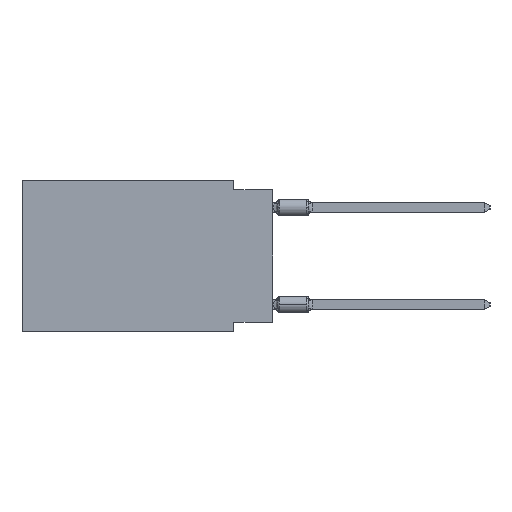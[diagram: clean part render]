
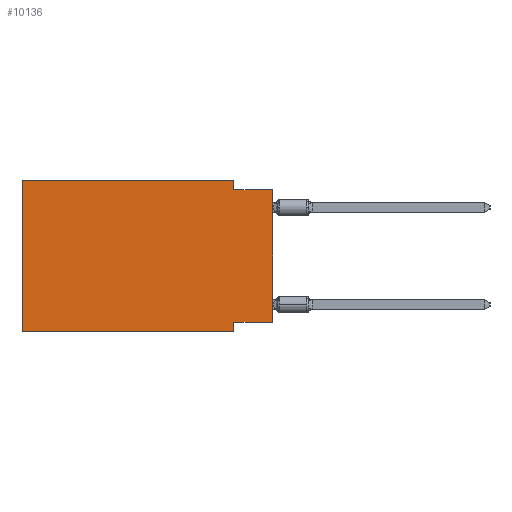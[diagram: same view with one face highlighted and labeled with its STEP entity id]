
A CAD part, left-side view. The second image highlights one B-rep face of the part: STEP entity #10136.
In plain terms, the highlighted planar face has unit normal (-1, 0, 0).
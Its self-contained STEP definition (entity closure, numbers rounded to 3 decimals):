
#2403 = EDGE_CURVE ( 'NONE', #34300, #35724, #3227, .T. ) ;
#3074 = PLANE ( 'NONE',  #36051 ) ;
#3227 = LINE ( 'NONE', #15440, #22596 ) ;
#3303 = VERTEX_POINT ( 'NONE', #22707 ) ;
#3503 = ORIENTED_EDGE ( 'NONE', *, *, #7575, .F. ) ;
#4296 = CARTESIAN_POINT ( 'NONE',  ( 0., 0., -0.635 ) ) ;
#6061 = VECTOR ( 'NONE', #17553, 1000. ) ;
#7575 = EDGE_CURVE ( 'NONE', #7789, #28297, #34504, .T. ) ;
#7760 = DIRECTION ( 'NONE',  ( 0., 1., 0. ) ) ;
#7789 = VERTEX_POINT ( 'NONE', #24601 ) ;
#9478 = DIRECTION ( 'NONE',  ( 0., 0., -1. ) ) ;
#10136 = ADVANCED_FACE ( 'NONE', ( #36728 ), #3074, .F. ) ;
#10223 = VECTOR ( 'NONE', #7760, 1000. ) ;
#11409 = CARTESIAN_POINT ( 'NONE',  ( 0., 0., 0. ) ) ;
#11563 = ORIENTED_EDGE ( 'NONE', *, *, #27276, .F. ) ;
#11667 = VECTOR ( 'NONE', #11803, 1000. ) ;
#11803 = DIRECTION ( 'NONE',  ( 0., 0., 1. ) ) ;
#13153 = ORIENTED_EDGE ( 'NONE', *, *, #30991, .F. ) ;
#14601 = DIRECTION ( 'NONE',  ( 0., -1., 0. ) ) ;
#15440 = CARTESIAN_POINT ( 'NONE',  ( 0., 16.383, 0. ) ) ;
#17553 = DIRECTION ( 'NONE',  ( 0., 0., 1. ) ) ;
#17715 = DIRECTION ( 'NONE',  ( 0., 0., -1. ) ) ;
#17812 = LINE ( 'NONE', #11409, #11667 ) ;
#18923 = CARTESIAN_POINT ( 'NONE',  ( 0., 16.383, -9.906 ) ) ;
#19049 = EDGE_CURVE ( 'NONE', #3303, #7789, #28595, .T. ) ;
#19502 = CARTESIAN_POINT ( 'NONE',  ( 0., 2.54, -9.906 ) ) ;
#19575 = CARTESIAN_POINT ( 'NONE',  ( 0., 0., -9.271 ) ) ;
#20283 = CARTESIAN_POINT ( 'NONE',  ( 0., 16.383, 0. ) ) ;
#20341 = ORIENTED_EDGE ( 'NONE', *, *, #38689, .T. ) ;
#21105 = CARTESIAN_POINT ( 'NONE',  ( 0., 16.383, 0. ) ) ;
#21248 = EDGE_CURVE ( 'NONE', #29459, #31257, #23619, .T. ) ;
#21683 = CARTESIAN_POINT ( 'NONE',  ( 0., 2.54, -9.906 ) ) ;
#22413 = EDGE_CURVE ( 'NONE', #3303, #31257, #17812, .T. ) ;
#22596 = VECTOR ( 'NONE', #36303, 1000. ) ;
#22707 = CARTESIAN_POINT ( 'NONE',  ( 0., 0., -9.271 ) ) ;
#23619 = LINE ( 'NONE', #35842, #27612 ) ;
#23967 = CARTESIAN_POINT ( 'NONE',  ( 0., 16.383, 0. ) ) ;
#24601 = CARTESIAN_POINT ( 'NONE',  ( 0., 2.54, -9.271 ) ) ;
#25936 = VERTEX_POINT ( 'NONE', #34631 ) ;
#26079 = CARTESIAN_POINT ( 'NONE',  ( 0., 2.54, 0. ) ) ;
#26273 = DIRECTION ( 'NONE',  ( 0., 0., -1. ) ) ;
#26600 = VECTOR ( 'NONE', #9478, 1000. ) ;
#26767 = LINE ( 'NONE', #18923, #34926 ) ;
#27276 = EDGE_CURVE ( 'NONE', #35724, #29459, #34892, .T. ) ;
#27612 = VECTOR ( 'NONE', #14601, 1000. ) ;
#27640 = ORIENTED_EDGE ( 'NONE', *, *, #2403, .F. ) ;
#28297 = VERTEX_POINT ( 'NONE', #19502 ) ;
#28595 = LINE ( 'NONE', #19575, #10223 ) ;
#28654 = ORIENTED_EDGE ( 'NONE', *, *, #22413, .T. ) ;
#29389 = ORIENTED_EDGE ( 'NONE', *, *, #21248, .F. ) ;
#29459 = VERTEX_POINT ( 'NONE', #30021 ) ;
#30021 = CARTESIAN_POINT ( 'NONE',  ( 0., 2.54, -0.635 ) ) ;
#30951 = DIRECTION ( 'NONE',  ( 0., -1., 0. ) ) ;
#30991 = EDGE_CURVE ( 'NONE', #25936, #34300, #36766, .T. ) ;
#31257 = VERTEX_POINT ( 'NONE', #4296 ) ;
#33527 = DIRECTION ( 'NONE',  ( 1., 0., 0. ) ) ;
#34300 = VERTEX_POINT ( 'NONE', #20283 ) ;
#34504 = LINE ( 'NONE', #21683, #26600 ) ;
#34631 = CARTESIAN_POINT ( 'NONE',  ( 0., 16.383, -9.906 ) ) ;
#34892 = LINE ( 'NONE', #26079, #37302 ) ;
#34926 = VECTOR ( 'NONE', #30951, 1000. ) ;
#35724 = VERTEX_POINT ( 'NONE', #37093 ) ;
#35842 = CARTESIAN_POINT ( 'NONE',  ( 0., 0., -0.635 ) ) ;
#36051 = AXIS2_PLACEMENT_3D ( 'NONE', #21105, #33527, #17715 ) ;
#36303 = DIRECTION ( 'NONE',  ( 0., -1., 0. ) ) ;
#36728 = FACE_OUTER_BOUND ( 'NONE', #37600, .T. ) ;
#36766 = LINE ( 'NONE', #23967, #6061 ) ;
#37093 = CARTESIAN_POINT ( 'NONE',  ( 0., 2.54, 0. ) ) ;
#37302 = VECTOR ( 'NONE', #26273, 1000. ) ;
#37600 = EDGE_LOOP ( 'NONE', ( #28654, #29389, #11563, #27640, #13153, #20341, #3503, #38086 ) ) ;
#38086 = ORIENTED_EDGE ( 'NONE', *, *, #19049, .F. ) ;
#38689 = EDGE_CURVE ( 'NONE', #25936, #28297, #26767, .T. ) ;
